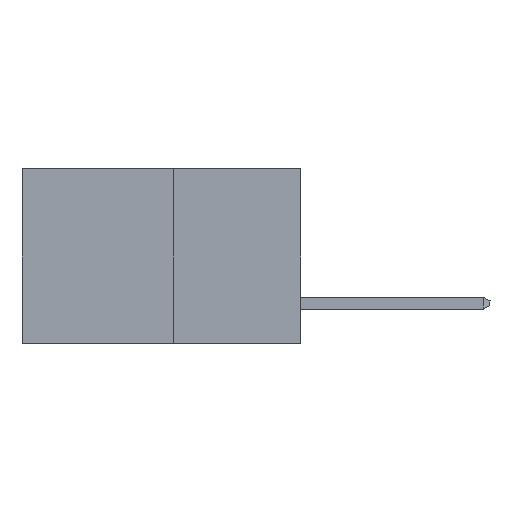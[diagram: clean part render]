
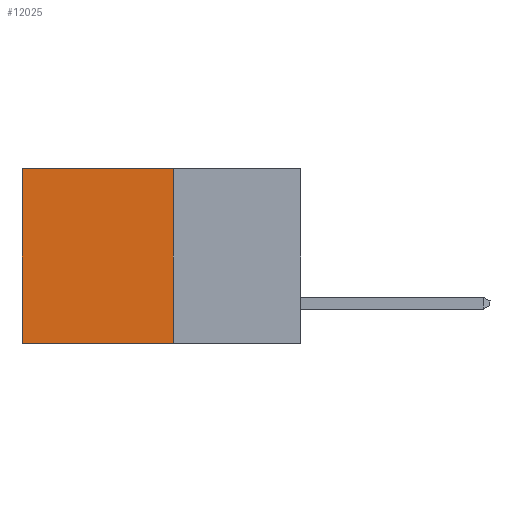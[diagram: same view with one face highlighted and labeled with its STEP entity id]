
A CAD part, left-side view. The second image highlights one B-rep face of the part: STEP entity #12025.
In plain terms, the highlighted planar face has unit normal (-1, 0, 0).
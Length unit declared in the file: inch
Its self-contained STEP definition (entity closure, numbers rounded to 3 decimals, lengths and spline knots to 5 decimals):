
#531 = CARTESIAN_POINT ( 'NONE',  ( 0.277, 0.59, 0. ) ) ;
#2352 = VECTOR ( 'NONE', #3061, 39.37008 ) ;
#2513 = DIRECTION ( 'NONE',  ( 0., 0., -1. ) ) ;
#2558 = LINE ( 'NONE', #13567, #13462 ) ;
#2578 = EDGE_CURVE ( 'NONE', #14685, #6749, #13540, .T. ) ;
#2813 = LINE ( 'NONE', #10914, #2352 ) ;
#3061 = DIRECTION ( 'NONE',  ( 0., 0., -1. ) ) ;
#3062 = CARTESIAN_POINT ( 'NONE',  ( 0.277, 0.27, 0. ) ) ;
#4155 = EDGE_CURVE ( 'NONE', #9112, #12507, #2813, .T. ) ;
#4269 = AXIS2_PLACEMENT_3D ( 'NONE', #16272, #7970, #17687 ) ;
#5069 = PLANE ( 'NONE',  #4269 ) ;
#5419 = CARTESIAN_POINT ( 'NONE',  ( 0.277, 0.59, -0.37 ) ) ;
#6749 = VERTEX_POINT ( 'NONE', #12671 ) ;
#6940 = CARTESIAN_POINT ( 'NONE',  ( 0.277, 0.27, 0. ) ) ;
#7332 = ORIENTED_EDGE ( 'NONE', *, *, #11450, .F. ) ;
#7970 = DIRECTION ( 'NONE',  ( 1., 0., 0. ) ) ;
#8942 = ORIENTED_EDGE ( 'NONE', *, *, #4155, .F. ) ;
#9112 = VERTEX_POINT ( 'NONE', #6940 ) ;
#9606 = ORIENTED_EDGE ( 'NONE', *, *, #2578, .T. ) ;
#10531 = VECTOR ( 'NONE', #14388, 39.37008 ) ;
#10914 = CARTESIAN_POINT ( 'NONE',  ( 0.277, 0.27, -0.37 ) ) ;
#11450 = EDGE_CURVE ( 'NONE', #12507, #6749, #2558, .T. ) ;
#12025 = ADVANCED_FACE ( 'NONE', ( #14073 ), #5069, .F. ) ;
#12507 = VERTEX_POINT ( 'NONE', #14751 ) ;
#12671 = CARTESIAN_POINT ( 'NONE',  ( 0.277, 0.59, -0.37 ) ) ;
#13462 = VECTOR ( 'NONE', #14904, 39.37008 ) ;
#13540 = LINE ( 'NONE', #5419, #17246 ) ;
#13567 = CARTESIAN_POINT ( 'NONE',  ( 0.277, 0.27, -0.37 ) ) ;
#13634 = EDGE_CURVE ( 'NONE', #9112, #14685, #14156, .T. ) ;
#13726 = ORIENTED_EDGE ( 'NONE', *, *, #13634, .T. ) ;
#14073 = FACE_OUTER_BOUND ( 'NONE', #15931, .T. ) ;
#14156 = LINE ( 'NONE', #3062, #10531 ) ;
#14388 = DIRECTION ( 'NONE',  ( 0., 1., 0. ) ) ;
#14685 = VERTEX_POINT ( 'NONE', #531 ) ;
#14751 = CARTESIAN_POINT ( 'NONE',  ( 0.277, 0.27, -0.37 ) ) ;
#14904 = DIRECTION ( 'NONE',  ( 0., 1., 0. ) ) ;
#15931 = EDGE_LOOP ( 'NONE', ( #9606, #7332, #8942, #13726 ) ) ;
#16272 = CARTESIAN_POINT ( 'NONE',  ( 0.277, 0.27, -0.37 ) ) ;
#17246 = VECTOR ( 'NONE', #2513, 39.37008 ) ;
#17687 = DIRECTION ( 'NONE',  ( 0., 0., -1. ) ) ;
